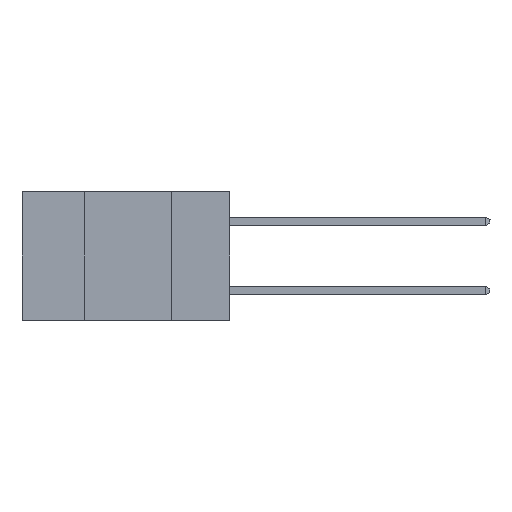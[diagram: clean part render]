
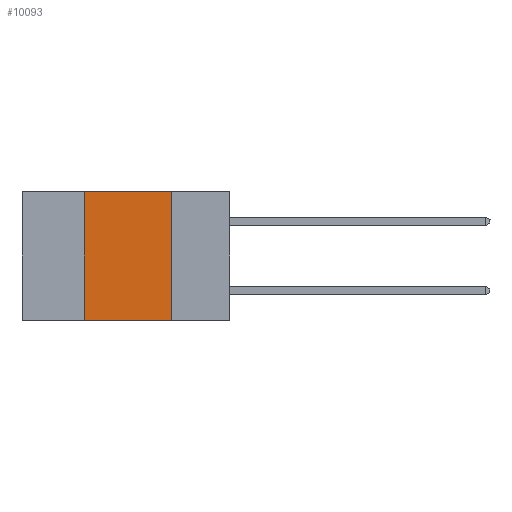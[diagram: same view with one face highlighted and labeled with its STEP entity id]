
A CAD part, left-side view. The second image highlights one B-rep face of the part: STEP entity #10093.
In plain terms, the highlighted planar face has unit normal (-1, 0, 0).
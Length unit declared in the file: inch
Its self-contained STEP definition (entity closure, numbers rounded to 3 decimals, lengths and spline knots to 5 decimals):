
#51 = FACE_OUTER_BOUND ( 'NONE', #6938, .T. ) ;
#715 = LINE ( 'NONE', #5432, #19350 ) ;
#1004 = EDGE_CURVE ( 'NONE', #3713, #19717, #18952, .T. ) ;
#1281 = VECTOR ( 'NONE', #7953, 39.37008 ) ;
#2328 = ORIENTED_EDGE ( 'NONE', *, *, #9656, .T. ) ;
#3125 = VECTOR ( 'NONE', #19915, 39.37008 ) ;
#3320 = CARTESIAN_POINT ( 'NONE',  ( 0., 0.42, -0.37 ) ) ;
#3713 = VERTEX_POINT ( 'NONE', #17646 ) ;
#4592 = LINE ( 'NONE', #18788, #3125 ) ;
#4996 = CARTESIAN_POINT ( 'NONE',  ( 0., 0.17, 0. ) ) ;
#5138 = DIRECTION ( 'NONE',  ( 0., 0., -1. ) ) ;
#5432 = CARTESIAN_POINT ( 'NONE',  ( 0., 0.6, 0. ) ) ;
#6164 = VERTEX_POINT ( 'NONE', #18199 ) ;
#6671 = EDGE_CURVE ( 'NONE', #19717, #6903, #715, .T. ) ;
#6903 = VERTEX_POINT ( 'NONE', #4996 ) ;
#6938 = EDGE_LOOP ( 'NONE', ( #18090, #11766, #12194, #2328 ) ) ;
#7458 = PLANE ( 'NONE',  #16154 ) ;
#7953 = DIRECTION ( 'NONE',  ( 0., 0., 1. ) ) ;
#9656 = EDGE_CURVE ( 'NONE', #3713, #6164, #4592, .T. ) ;
#9680 = DIRECTION ( 'NONE',  ( 1., 0., 0. ) ) ;
#10093 = ADVANCED_FACE ( 'NONE', ( #51 ), #7458, .F. ) ;
#10986 = CARTESIAN_POINT ( 'NONE',  ( 0., 0.6, 0. ) ) ;
#11766 = ORIENTED_EDGE ( 'NONE', *, *, #6671, .F. ) ;
#12194 = ORIENTED_EDGE ( 'NONE', *, *, #1004, .F. ) ;
#12681 = LINE ( 'NONE', #12781, #18565 ) ;
#12781 = CARTESIAN_POINT ( 'NONE',  ( 0., 0.17, -0.37 ) ) ;
#13268 = DIRECTION ( 'NONE',  ( 0., -1., 0. ) ) ;
#13549 = DIRECTION ( 'NONE',  ( 0., 0., -1. ) ) ;
#13614 = EDGE_CURVE ( 'NONE', #6903, #6164, #12681, .T. ) ;
#16154 = AXIS2_PLACEMENT_3D ( 'NONE', #10986, #9680, #13549 ) ;
#17326 = CARTESIAN_POINT ( 'NONE',  ( 0., 0.42, 0. ) ) ;
#17646 = CARTESIAN_POINT ( 'NONE',  ( 0., 0.42, -0.37 ) ) ;
#18090 = ORIENTED_EDGE ( 'NONE', *, *, #13614, .F. ) ;
#18199 = CARTESIAN_POINT ( 'NONE',  ( 0., 0.17, -0.37 ) ) ;
#18565 = VECTOR ( 'NONE', #5138, 39.37008 ) ;
#18788 = CARTESIAN_POINT ( 'NONE',  ( 0., 0.6, -0.37 ) ) ;
#18952 = LINE ( 'NONE', #3320, #1281 ) ;
#19350 = VECTOR ( 'NONE', #13268, 39.37008 ) ;
#19717 = VERTEX_POINT ( 'NONE', #17326 ) ;
#19915 = DIRECTION ( 'NONE',  ( 0., -1., 0. ) ) ;
